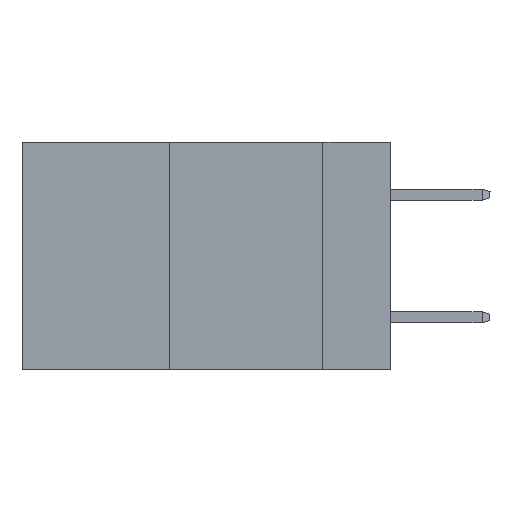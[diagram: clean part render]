
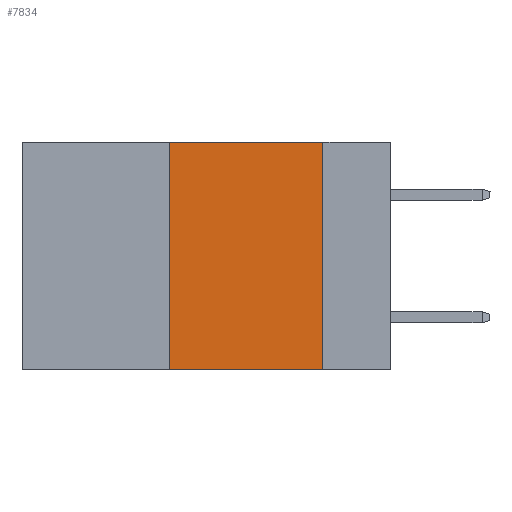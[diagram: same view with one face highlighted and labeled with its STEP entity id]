
A CAD part, left-side view. The second image highlights one B-rep face of the part: STEP entity #7834.
In plain terms, the highlighted planar face has unit normal (-1, 0, 0).
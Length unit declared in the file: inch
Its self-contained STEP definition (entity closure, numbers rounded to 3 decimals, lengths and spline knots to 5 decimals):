
#554 = CARTESIAN_POINT ( 'NONE',  ( 0., 0.6, -0.37 ) ) ;
#1163 = ORIENTED_EDGE ( 'NONE', *, *, #1637, .F. ) ;
#1637 = EDGE_CURVE ( 'NONE', #6826, #12926, #6278, .T. ) ;
#2030 = DIRECTION ( 'NONE',  ( 0., -1., 0. ) ) ;
#2167 = EDGE_CURVE ( 'NONE', #4413, #6380, #13801, .T. ) ;
#2378 = CARTESIAN_POINT ( 'NONE',  ( 0., 0.36, 0. ) ) ;
#4159 = EDGE_CURVE ( 'NONE', #4413, #12926, #13952, .T. ) ;
#4180 = CARTESIAN_POINT ( 'NONE',  ( 0., 0.11, 0. ) ) ;
#4183 = DIRECTION ( 'NONE',  ( 0., -1., 0. ) ) ;
#4413 = VERTEX_POINT ( 'NONE', #5857 ) ;
#4590 = ORIENTED_EDGE ( 'NONE', *, *, #4159, .T. ) ;
#5116 = VECTOR ( 'NONE', #11699, 39.37008 ) ;
#5857 = CARTESIAN_POINT ( 'NONE',  ( 0., 0.36, -0.37 ) ) ;
#6278 = LINE ( 'NONE', #4180, #5116 ) ;
#6380 = VERTEX_POINT ( 'NONE', #10182 ) ;
#6826 = VERTEX_POINT ( 'NONE', #13465 ) ;
#7236 = EDGE_CURVE ( 'NONE', #6380, #6826, #17872, .T. ) ;
#7647 = ORIENTED_EDGE ( 'NONE', *, *, #2167, .F. ) ;
#7834 = ADVANCED_FACE ( 'NONE', ( #16882 ), #16242, .F. ) ;
#8432 = VECTOR ( 'NONE', #4183, 39.37008 ) ;
#8509 = DIRECTION ( 'NONE',  ( 0., 0., 1. ) ) ;
#8662 = DIRECTION ( 'NONE',  ( 1., 0., 0. ) ) ;
#10014 = EDGE_LOOP ( 'NONE', ( #1163, #10033, #7647, #4590 ) ) ;
#10033 = ORIENTED_EDGE ( 'NONE', *, *, #7236, .F. ) ;
#10182 = CARTESIAN_POINT ( 'NONE',  ( 0., 0.36, 0. ) ) ;
#11521 = DIRECTION ( 'NONE',  ( 0., 0., -1. ) ) ;
#11699 = DIRECTION ( 'NONE',  ( 0., 0., -1. ) ) ;
#11724 = CARTESIAN_POINT ( 'NONE',  ( 0., 0.6, 0. ) ) ;
#12692 = CARTESIAN_POINT ( 'NONE',  ( 0., 0.11, -0.37 ) ) ;
#12924 = AXIS2_PLACEMENT_3D ( 'NONE', #11724, #8662, #11521 ) ;
#12926 = VERTEX_POINT ( 'NONE', #12692 ) ;
#13465 = CARTESIAN_POINT ( 'NONE',  ( 0., 0.11, 0. ) ) ;
#13801 = LINE ( 'NONE', #2378, #15448 ) ;
#13952 = LINE ( 'NONE', #554, #16348 ) ;
#15448 = VECTOR ( 'NONE', #8509, 39.37008 ) ;
#16242 = PLANE ( 'NONE',  #12924 ) ;
#16348 = VECTOR ( 'NONE', #2030, 39.37008 ) ;
#16882 = FACE_OUTER_BOUND ( 'NONE', #10014, .T. ) ;
#17791 = CARTESIAN_POINT ( 'NONE',  ( 0., 0.6, 0. ) ) ;
#17872 = LINE ( 'NONE', #17791, #8432 ) ;
